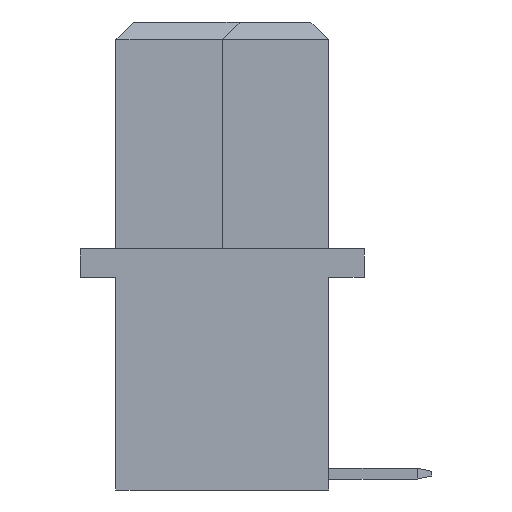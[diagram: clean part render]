
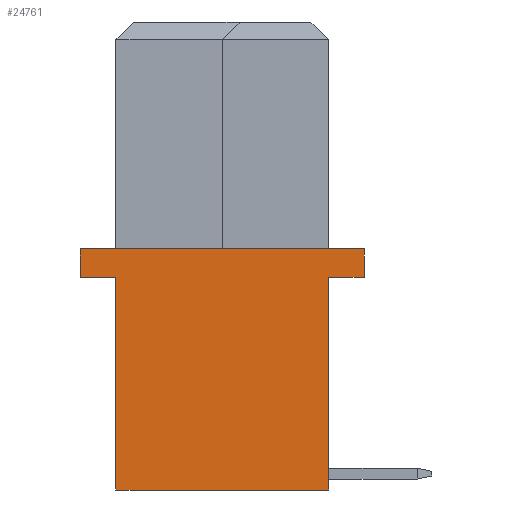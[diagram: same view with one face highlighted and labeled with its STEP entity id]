
A CAD part, left-side view. The second image highlights one B-rep face of the part: STEP entity #24761.
In plain terms, the highlighted planar face has unit normal (-1, 0, 0).
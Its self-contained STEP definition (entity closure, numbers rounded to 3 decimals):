
#246 = DIRECTION ( 'NONE',  ( 0., 0., -1. ) ) ;
#891 = LINE ( 'NONE', #13134, #14211 ) ;
#959 = AXIS2_PLACEMENT_3D ( 'NONE', #1172, #15717, #7635 ) ;
#1017 = ORIENTED_EDGE ( 'NONE', *, *, #3990, .F. ) ;
#1172 = CARTESIAN_POINT ( 'NONE',  ( -47., -4., -13.2 ) ) ;
#2200 = EDGE_CURVE ( 'NONE', #22453, #17073, #18823, .T. ) ;
#2605 = EDGE_LOOP ( 'NONE', ( #18083, #1017, #23871, #14833, #14864, #6232, #23227, #13644 ) ) ;
#2710 = EDGE_CURVE ( 'NONE', #17073, #19650, #891, .T. ) ;
#3149 = VERTEX_POINT ( 'NONE', #4767 ) ;
#3304 = DIRECTION ( 'NONE',  ( 0., 0., 1. ) ) ;
#3990 = EDGE_CURVE ( 'NONE', #19329, #12230, #6965, .T. ) ;
#4048 = CARTESIAN_POINT ( 'NONE',  ( -47., 3., -7.2 ) ) ;
#4348 = LINE ( 'NONE', #20644, #6954 ) ;
#4736 = EDGE_CURVE ( 'NONE', #19329, #16612, #4348, .T. ) ;
#4767 = CARTESIAN_POINT ( 'NONE',  ( -47., -3., -13.2 ) ) ;
#4779 = DIRECTION ( 'NONE',  ( 0., 0., -1. ) ) ;
#5589 = EDGE_CURVE ( 'NONE', #24774, #3149, #14598, .T. ) ;
#5655 = VECTOR ( 'NONE', #16140, 1000. ) ;
#5966 = CARTESIAN_POINT ( 'NONE',  ( -47., 3., -7.2 ) ) ;
#6000 = VECTOR ( 'NONE', #9236, 1000. ) ;
#6188 = CARTESIAN_POINT ( 'NONE',  ( -47., 4., -6.4 ) ) ;
#6232 = ORIENTED_EDGE ( 'NONE', *, *, #2200, .F. ) ;
#6954 = VECTOR ( 'NONE', #12281, 1000. ) ;
#6965 = LINE ( 'NONE', #9506, #6000 ) ;
#7635 = DIRECTION ( 'NONE',  ( 0., 0., 1. ) ) ;
#7946 = LINE ( 'NONE', #6188, #5655 ) ;
#8852 = CARTESIAN_POINT ( 'NONE',  ( -47., -3., -7.2 ) ) ;
#9236 = DIRECTION ( 'NONE',  ( 0., 1., 0. ) ) ;
#9506 = CARTESIAN_POINT ( 'NONE',  ( -47., -3., -7.2 ) ) ;
#10694 = CARTESIAN_POINT ( 'NONE',  ( -47., -4., -13.2 ) ) ;
#12065 = EDGE_CURVE ( 'NONE', #19650, #16612, #7946, .T. ) ;
#12230 = VERTEX_POINT ( 'NONE', #8852 ) ;
#12281 = DIRECTION ( 'NONE',  ( 0., 0., 1. ) ) ;
#13134 = CARTESIAN_POINT ( 'NONE',  ( -47., 4., -13.2 ) ) ;
#13644 = ORIENTED_EDGE ( 'NONE', *, *, #5589, .T. ) ;
#14211 = VECTOR ( 'NONE', #3304, 1000. ) ;
#14598 = LINE ( 'NONE', #10694, #23622 ) ;
#14833 = ORIENTED_EDGE ( 'NONE', *, *, #12065, .F. ) ;
#14859 = DIRECTION ( 'NONE',  ( 0., -1., 0. ) ) ;
#14864 = ORIENTED_EDGE ( 'NONE', *, *, #2710, .F. ) ;
#15389 = CARTESIAN_POINT ( 'NONE',  ( -47., -4., -7.2 ) ) ;
#15717 = DIRECTION ( 'NONE',  ( -1., 0., 0. ) ) ;
#16140 = DIRECTION ( 'NONE',  ( 0., -1., 0. ) ) ;
#16608 = CARTESIAN_POINT ( 'NONE',  ( -47., -4., -6.4 ) ) ;
#16612 = VERTEX_POINT ( 'NONE', #16608 ) ;
#16659 = CARTESIAN_POINT ( 'NONE',  ( -47., 4., -7.2 ) ) ;
#16898 = VECTOR ( 'NONE', #4779, 1000. ) ;
#17073 = VERTEX_POINT ( 'NONE', #19786 ) ;
#17469 = PLANE ( 'NONE',  #959 ) ;
#17605 = FACE_OUTER_BOUND ( 'NONE', #2605, .T. ) ;
#18083 = ORIENTED_EDGE ( 'NONE', *, *, #26361, .F. ) ;
#18518 = VECTOR ( 'NONE', #246, 1000. ) ;
#18823 = LINE ( 'NONE', #16659, #25888 ) ;
#19329 = VERTEX_POINT ( 'NONE', #15389 ) ;
#19590 = CARTESIAN_POINT ( 'NONE',  ( -47., -3., -7.2 ) ) ;
#19650 = VERTEX_POINT ( 'NONE', #26445 ) ;
#19786 = CARTESIAN_POINT ( 'NONE',  ( -47., 4., -7.2 ) ) ;
#19868 = EDGE_CURVE ( 'NONE', #22453, #24774, #22508, .T. ) ;
#20030 = CARTESIAN_POINT ( 'NONE',  ( -47., 3., -13.2 ) ) ;
#20644 = CARTESIAN_POINT ( 'NONE',  ( -47., -4., -13.2 ) ) ;
#22453 = VERTEX_POINT ( 'NONE', #5966 ) ;
#22508 = LINE ( 'NONE', #4048, #18518 ) ;
#23023 = DIRECTION ( 'NONE',  ( 0., 1., 0. ) ) ;
#23227 = ORIENTED_EDGE ( 'NONE', *, *, #19868, .T. ) ;
#23238 = LINE ( 'NONE', #19590, #16898 ) ;
#23622 = VECTOR ( 'NONE', #14859, 1000. ) ;
#23871 = ORIENTED_EDGE ( 'NONE', *, *, #4736, .T. ) ;
#24761 = ADVANCED_FACE ( 'NONE', ( #17605 ), #17469, .T. ) ;
#24774 = VERTEX_POINT ( 'NONE', #20030 ) ;
#25888 = VECTOR ( 'NONE', #23023, 1000. ) ;
#26361 = EDGE_CURVE ( 'NONE', #12230, #3149, #23238, .T. ) ;
#26445 = CARTESIAN_POINT ( 'NONE',  ( -47., 4., -6.4 ) ) ;
